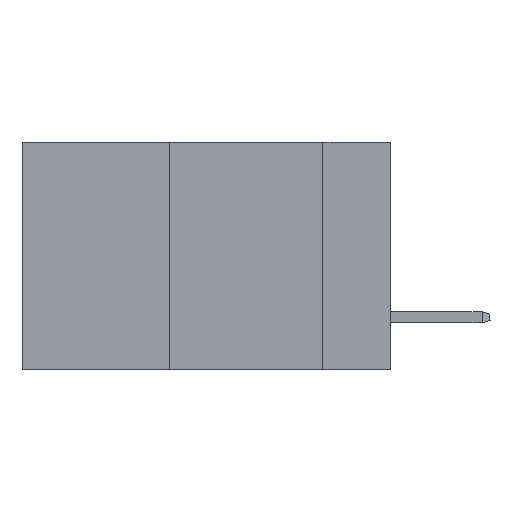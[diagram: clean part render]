
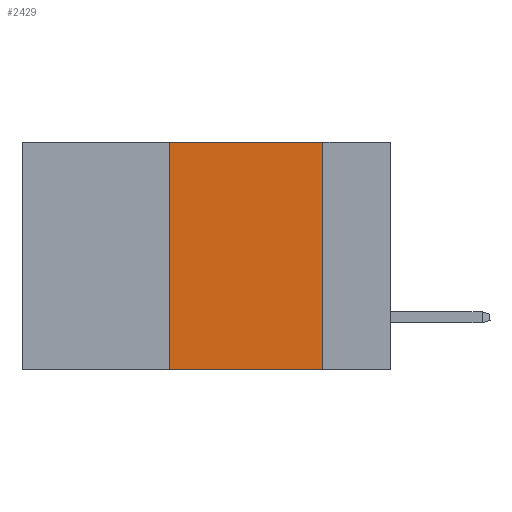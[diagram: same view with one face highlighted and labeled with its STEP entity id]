
A CAD part, left-side view. The second image highlights one B-rep face of the part: STEP entity #2429.
In plain terms, the highlighted planar face has unit normal (-1, 0, 0).
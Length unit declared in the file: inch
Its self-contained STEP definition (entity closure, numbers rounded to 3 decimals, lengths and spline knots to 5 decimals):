
#1481 = LINE ( 'NONE', #19609, #20426 ) ;
#2209 = VERTEX_POINT ( 'NONE', #10069 ) ;
#2429 = ADVANCED_FACE ( 'NONE', ( #15344 ), #24791, .F. ) ;
#2672 = ORIENTED_EDGE ( 'NONE', *, *, #18948, .F. ) ;
#3108 = CARTESIAN_POINT ( 'NONE',  ( 0., 0.36, -0.37 ) ) ;
#3787 = ORIENTED_EDGE ( 'NONE', *, *, #16241, .F. ) ;
#3974 = EDGE_CURVE ( 'NONE', #6314, #18179, #1481, .T. ) ;
#4593 = DIRECTION ( 'NONE',  ( 1., 0., 0. ) ) ;
#4647 = CARTESIAN_POINT ( 'NONE',  ( 0., 0.11, -0.37 ) ) ;
#5693 = CARTESIAN_POINT ( 'NONE',  ( 0., 0.6, 0. ) ) ;
#6314 = VERTEX_POINT ( 'NONE', #3108 ) ;
#6875 = VERTEX_POINT ( 'NONE', #4647 ) ;
#8033 = CARTESIAN_POINT ( 'NONE',  ( 0., 0.6, -0.37 ) ) ;
#8551 = EDGE_CURVE ( 'NONE', #6314, #6875, #28234, .T. ) ;
#8576 = DIRECTION ( 'NONE',  ( 0., 0., -1. ) ) ;
#9544 = VECTOR ( 'NONE', #24378, 39.37008 ) ;
#10069 = CARTESIAN_POINT ( 'NONE',  ( 0., 0.11, 0. ) ) ;
#10115 = LINE ( 'NONE', #5693, #23621 ) ;
#10710 = ORIENTED_EDGE ( 'NONE', *, *, #8551, .T. ) ;
#13339 = ORIENTED_EDGE ( 'NONE', *, *, #3974, .F. ) ;
#13484 = LINE ( 'NONE', #15704, #14298 ) ;
#13941 = AXIS2_PLACEMENT_3D ( 'NONE', #18147, #4593, #8576 ) ;
#14298 = VECTOR ( 'NONE', #24709, 39.37008 ) ;
#15250 = EDGE_LOOP ( 'NONE', ( #2672, #3787, #13339, #10710 ) ) ;
#15344 = FACE_OUTER_BOUND ( 'NONE', #15250, .T. ) ;
#15704 = CARTESIAN_POINT ( 'NONE',  ( 0., 0.11, 0. ) ) ;
#16241 = EDGE_CURVE ( 'NONE', #18179, #2209, #10115, .T. ) ;
#16584 = DIRECTION ( 'NONE',  ( 0., -1., 0. ) ) ;
#17153 = CARTESIAN_POINT ( 'NONE',  ( 0., 0.36, 0. ) ) ;
#18147 = CARTESIAN_POINT ( 'NONE',  ( 0., 0.6, 0. ) ) ;
#18179 = VERTEX_POINT ( 'NONE', #17153 ) ;
#18948 = EDGE_CURVE ( 'NONE', #2209, #6875, #13484, .T. ) ;
#19032 = DIRECTION ( 'NONE',  ( 0., 0., 1. ) ) ;
#19609 = CARTESIAN_POINT ( 'NONE',  ( 0., 0.36, 0. ) ) ;
#20426 = VECTOR ( 'NONE', #19032, 39.37008 ) ;
#23621 = VECTOR ( 'NONE', #16584, 39.37008 ) ;
#24378 = DIRECTION ( 'NONE',  ( 0., -1., 0. ) ) ;
#24709 = DIRECTION ( 'NONE',  ( 0., 0., -1. ) ) ;
#24791 = PLANE ( 'NONE',  #13941 ) ;
#28234 = LINE ( 'NONE', #8033, #9544 ) ;
